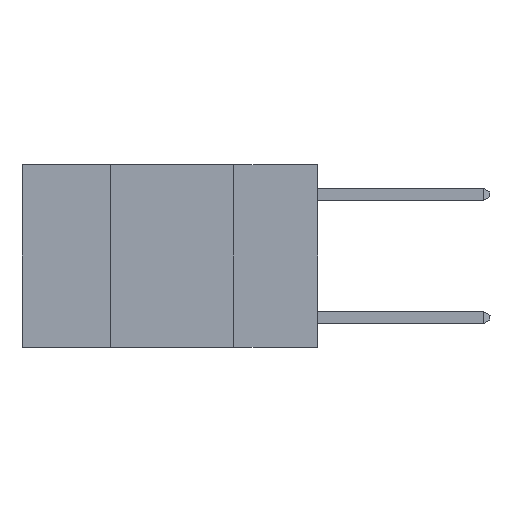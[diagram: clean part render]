
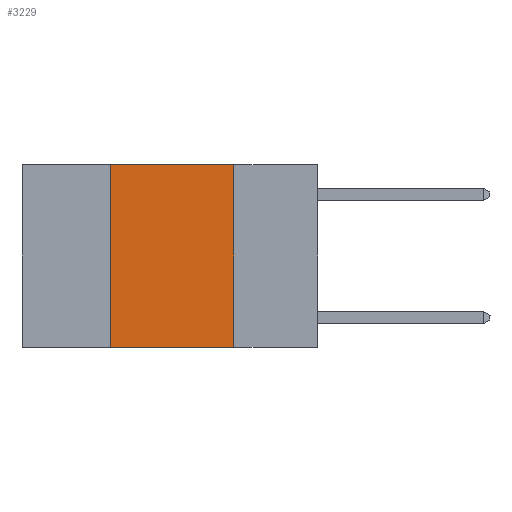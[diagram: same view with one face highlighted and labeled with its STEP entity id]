
A CAD part, left-side view. The second image highlights one B-rep face of the part: STEP entity #3229.
In plain terms, the highlighted planar face has unit normal (-1, 0, 0).
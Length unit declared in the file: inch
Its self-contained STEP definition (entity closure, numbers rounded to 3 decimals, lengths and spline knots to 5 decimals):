
#1137 = ORIENTED_EDGE ( 'NONE', *, *, #23872, .F. ) ;
#2510 = CARTESIAN_POINT ( 'NONE',  ( 0., 0.42, -0.37 ) ) ;
#3177 = CARTESIAN_POINT ( 'NONE',  ( 0., 0.42, 0. ) ) ;
#3229 = ADVANCED_FACE ( 'NONE', ( #15307 ), #11088, .F. ) ;
#5121 = EDGE_CURVE ( 'NONE', #12975, #14129, #15959, .T. ) ;
#8825 = CARTESIAN_POINT ( 'NONE',  ( 0., 0.17, 0. ) ) ;
#9106 = DIRECTION ( 'NONE',  ( 0., -1., 0. ) ) ;
#9114 = VECTOR ( 'NONE', #17838, 39.37008 ) ;
#11088 = PLANE ( 'NONE',  #24166 ) ;
#12037 = ORIENTED_EDGE ( 'NONE', *, *, #21305, .F. ) ;
#12899 = EDGE_LOOP ( 'NONE', ( #12037, #25767, #1137, #21612 ) ) ;
#12975 = VERTEX_POINT ( 'NONE', #2510 ) ;
#13627 = DIRECTION ( 'NONE',  ( 1., 0., 0. ) ) ;
#14129 = VERTEX_POINT ( 'NONE', #26030 ) ;
#14966 = LINE ( 'NONE', #29885, #9114 ) ;
#15307 = FACE_OUTER_BOUND ( 'NONE', #12899, .T. ) ;
#15959 = LINE ( 'NONE', #21386, #19390 ) ;
#16230 = DIRECTION ( 'NONE',  ( 0., 0., -1. ) ) ;
#17838 = DIRECTION ( 'NONE',  ( 0., -1., 0. ) ) ;
#18015 = CARTESIAN_POINT ( 'NONE',  ( 0., 0.42, 0. ) ) ;
#19390 = VECTOR ( 'NONE', #9106, 39.37008 ) ;
#21050 = EDGE_CURVE ( 'NONE', #29631, #27902, #14966, .T. ) ;
#21305 = EDGE_CURVE ( 'NONE', #27902, #14129, #30542, .T. ) ;
#21386 = CARTESIAN_POINT ( 'NONE',  ( 0., 0.6, -0.37 ) ) ;
#21612 = ORIENTED_EDGE ( 'NONE', *, *, #5121, .T. ) ;
#22839 = VECTOR ( 'NONE', #22854, 39.37008 ) ;
#22854 = DIRECTION ( 'NONE',  ( 0., 0., 1. ) ) ;
#23872 = EDGE_CURVE ( 'NONE', #12975, #29631, #29287, .T. ) ;
#24166 = AXIS2_PLACEMENT_3D ( 'NONE', #25731, #13627, #30602 ) ;
#25624 = VECTOR ( 'NONE', #16230, 39.37008 ) ;
#25731 = CARTESIAN_POINT ( 'NONE',  ( 0., 0.6, 0. ) ) ;
#25767 = ORIENTED_EDGE ( 'NONE', *, *, #21050, .F. ) ;
#26030 = CARTESIAN_POINT ( 'NONE',  ( 0., 0.17, -0.37 ) ) ;
#27902 = VERTEX_POINT ( 'NONE', #28842 ) ;
#28842 = CARTESIAN_POINT ( 'NONE',  ( 0., 0.17, 0. ) ) ;
#29287 = LINE ( 'NONE', #18015, #22839 ) ;
#29631 = VERTEX_POINT ( 'NONE', #3177 ) ;
#29885 = CARTESIAN_POINT ( 'NONE',  ( 0., 0.6, 0. ) ) ;
#30542 = LINE ( 'NONE', #8825, #25624 ) ;
#30602 = DIRECTION ( 'NONE',  ( 0., 0., -1. ) ) ;
